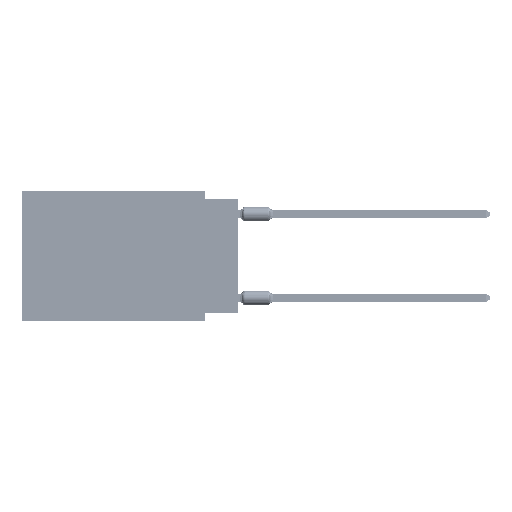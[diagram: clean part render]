
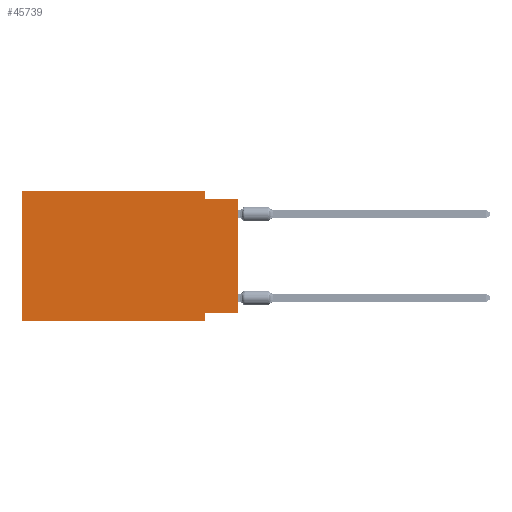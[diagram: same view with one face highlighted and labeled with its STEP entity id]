
A CAD part, left-side view. The second image highlights one B-rep face of the part: STEP entity #45739.
In plain terms, the highlighted planar face has unit normal (-1, 0, 0).
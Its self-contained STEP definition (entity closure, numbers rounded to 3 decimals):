
#814 = CARTESIAN_POINT ( 'NONE',  ( 0., 0., -9.271 ) ) ;
#1824 = AXIS2_PLACEMENT_3D ( 'NONE', #85740, #32325, #72923 ) ;
#2229 = ORIENTED_EDGE ( 'NONE', *, *, #73415, .F. ) ;
#3878 = VERTEX_POINT ( 'NONE', #32970 ) ;
#4205 = EDGE_LOOP ( 'NONE', ( #15039, #2229, #32634, #39436, #33999, #67794, #79822, #10312 ) ) ;
#4577 = CARTESIAN_POINT ( 'NONE',  ( 0., 0., 0. ) ) ;
#5702 = CARTESIAN_POINT ( 'NONE',  ( 0., 0., -0.635 ) ) ;
#7537 = LINE ( 'NONE', #34473, #68890 ) ;
#8822 = CARTESIAN_POINT ( 'NONE',  ( 0., 16.383, 0. ) ) ;
#10312 = ORIENTED_EDGE ( 'NONE', *, *, #31295, .F. ) ;
#11458 = VERTEX_POINT ( 'NONE', #80939 ) ;
#13002 = CARTESIAN_POINT ( 'NONE',  ( 0., 16.383, 0. ) ) ;
#13850 = LINE ( 'NONE', #65959, #66556 ) ;
#15039 = ORIENTED_EDGE ( 'NONE', *, *, #42678, .T. ) ;
#17308 = VECTOR ( 'NONE', #85654, 1000. ) ;
#17626 = EDGE_CURVE ( 'NONE', #76024, #11458, #54060, .T. ) ;
#20527 = VECTOR ( 'NONE', #74777, 1000. ) ;
#22836 = VECTOR ( 'NONE', #83514, 1000. ) ;
#23432 = CARTESIAN_POINT ( 'NONE',  ( 0., 2.54, -9.906 ) ) ;
#26537 = DIRECTION ( 'NONE',  ( 0., -1., 0. ) ) ;
#29302 = VERTEX_POINT ( 'NONE', #814 ) ;
#31295 = EDGE_CURVE ( 'NONE', #29302, #58849, #13850, .T. ) ;
#32325 = DIRECTION ( 'NONE',  ( 1., 0., 0. ) ) ;
#32375 = DIRECTION ( 'NONE',  ( 0., 0., 1. ) ) ;
#32634 = ORIENTED_EDGE ( 'NONE', *, *, #76435, .F. ) ;
#32970 = CARTESIAN_POINT ( 'NONE',  ( 0., 2.54, 0. ) ) ;
#33483 = VECTOR ( 'NONE', #62681, 1000. ) ;
#33999 = ORIENTED_EDGE ( 'NONE', *, *, #17626, .F. ) ;
#34473 = CARTESIAN_POINT ( 'NONE',  ( 0., 2.54, 0. ) ) ;
#34482 = CARTESIAN_POINT ( 'NONE',  ( 0., 0., -0.635 ) ) ;
#37111 = CARTESIAN_POINT ( 'NONE',  ( 0., 2.54, -9.271 ) ) ;
#37290 = VECTOR ( 'NONE', #32375, 1000. ) ;
#38566 = LINE ( 'NONE', #4577, #37290 ) ;
#39436 = ORIENTED_EDGE ( 'NONE', *, *, #75206, .F. ) ;
#42303 = CARTESIAN_POINT ( 'NONE',  ( 0., 2.54, -0.635 ) ) ;
#42678 = EDGE_CURVE ( 'NONE', #29302, #57818, #38566, .T. ) ;
#43719 = LINE ( 'NONE', #23432, #17308 ) ;
#45739 = ADVANCED_FACE ( 'NONE', ( #58824 ), #86149, .F. ) ;
#52709 = VERTEX_POINT ( 'NONE', #58271 ) ;
#54060 = LINE ( 'NONE', #13002, #20527 ) ;
#54666 = VECTOR ( 'NONE', #26537, 1000. ) ;
#57818 = VERTEX_POINT ( 'NONE', #5702 ) ;
#58271 = CARTESIAN_POINT ( 'NONE',  ( 0., 2.54, -9.906 ) ) ;
#58824 = FACE_OUTER_BOUND ( 'NONE', #4205, .T. ) ;
#58849 = VERTEX_POINT ( 'NONE', #37111 ) ;
#60093 = LINE ( 'NONE', #34482, #54666 ) ;
#61394 = DIRECTION ( 'NONE',  ( 0., 0., -1. ) ) ;
#62338 = LINE ( 'NONE', #81778, #22836 ) ;
#62681 = DIRECTION ( 'NONE',  ( 0., -1., 0. ) ) ;
#63234 = CARTESIAN_POINT ( 'NONE',  ( 0., 16.383, -9.906 ) ) ;
#65094 = EDGE_CURVE ( 'NONE', #76024, #52709, #62338, .T. ) ;
#65959 = CARTESIAN_POINT ( 'NONE',  ( 0., 0., -9.271 ) ) ;
#66556 = VECTOR ( 'NONE', #67688, 1000. ) ;
#67688 = DIRECTION ( 'NONE',  ( 0., 1., 0. ) ) ;
#67794 = ORIENTED_EDGE ( 'NONE', *, *, #65094, .T. ) ;
#68424 = LINE ( 'NONE', #8822, #33483 ) ;
#68890 = VECTOR ( 'NONE', #61394, 1000. ) ;
#72923 = DIRECTION ( 'NONE',  ( 0., 0., -1. ) ) ;
#73415 = EDGE_CURVE ( 'NONE', #83172, #57818, #60093, .T. ) ;
#74777 = DIRECTION ( 'NONE',  ( 0., 0., 1. ) ) ;
#75206 = EDGE_CURVE ( 'NONE', #11458, #3878, #68424, .T. ) ;
#76024 = VERTEX_POINT ( 'NONE', #63234 ) ;
#76435 = EDGE_CURVE ( 'NONE', #3878, #83172, #7537, .T. ) ;
#79822 = ORIENTED_EDGE ( 'NONE', *, *, #80408, .F. ) ;
#80408 = EDGE_CURVE ( 'NONE', #58849, #52709, #43719, .T. ) ;
#80939 = CARTESIAN_POINT ( 'NONE',  ( 0., 16.383, 0. ) ) ;
#81778 = CARTESIAN_POINT ( 'NONE',  ( 0., 16.383, -9.906 ) ) ;
#83172 = VERTEX_POINT ( 'NONE', #42303 ) ;
#83514 = DIRECTION ( 'NONE',  ( 0., -1., 0. ) ) ;
#85654 = DIRECTION ( 'NONE',  ( 0., 0., -1. ) ) ;
#85740 = CARTESIAN_POINT ( 'NONE',  ( 0., 16.383, 0. ) ) ;
#86149 = PLANE ( 'NONE',  #1824 ) ;
